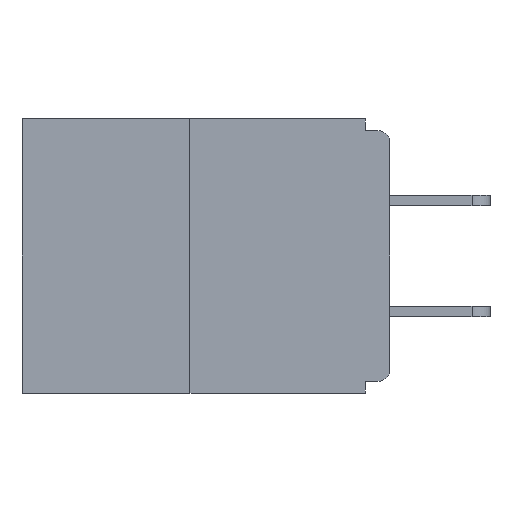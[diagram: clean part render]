
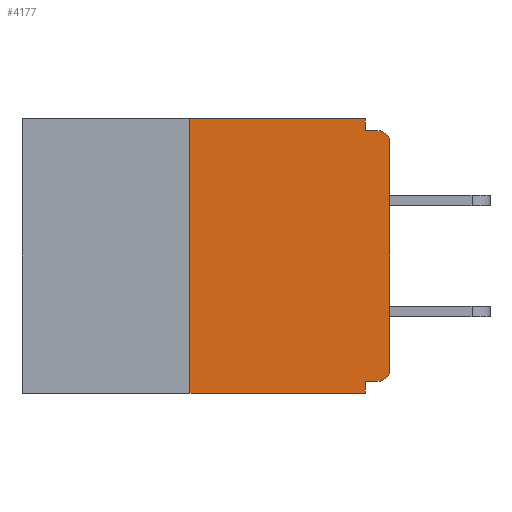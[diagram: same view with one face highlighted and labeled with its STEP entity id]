
A CAD part, left-side view. The second image highlights one B-rep face of the part: STEP entity #4177.
In plain terms, the highlighted planar face has unit normal (-1, 0, 0).
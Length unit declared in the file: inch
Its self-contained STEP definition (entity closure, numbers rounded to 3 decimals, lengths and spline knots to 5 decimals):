
#1193 = CARTESIAN_POINT ( 'NONE',  ( 0., 0., -0.03 ) ) ;
#1812 = ORIENTED_EDGE ( 'NONE', *, *, #10412, .F. ) ;
#1840 = CARTESIAN_POINT ( 'NONE',  ( 0., 0.015, -0.313 ) ) ;
#2341 = ORIENTED_EDGE ( 'NONE', *, *, #2377, .T. ) ;
#2377 = EDGE_CURVE ( 'NONE', #23291, #9017, #26616, .T. ) ;
#2640 = VERTEX_POINT ( 'NONE', #28057 ) ;
#2755 = CARTESIAN_POINT ( 'NONE',  ( 0., 0.015, -0.328 ) ) ;
#3317 = CARTESIAN_POINT ( 'NONE',  ( 0., 0., 0. ) ) ;
#4077 = EDGE_CURVE ( 'NONE', #2640, #22003, #6474, .T. ) ;
#4101 = VECTOR ( 'NONE', #17891, 39.37008 ) ;
#4158 = EDGE_CURVE ( 'NONE', #27172, #19350, #8565, .T. ) ;
#4177 = ADVANCED_FACE ( 'NONE', ( #21553 ), #20352, .F. ) ;
#4970 = DIRECTION ( 'NONE',  ( 1., 0., 0. ) ) ;
#5453 = AXIS2_PLACEMENT_3D ( 'NONE', #19837, #22134, #21942 ) ;
#5956 = CARTESIAN_POINT ( 'NONE',  ( 0., 0.031, -0.343 ) ) ;
#6432 = CARTESIAN_POINT ( 'NONE',  ( 0., 0.46, -0.343 ) ) ;
#6433 = CARTESIAN_POINT ( 'NONE',  ( 0., 0.25, -0.343 ) ) ;
#6474 = LINE ( 'NONE', #15413, #4101 ) ;
#6883 = VERTEX_POINT ( 'NONE', #27570 ) ;
#7820 = EDGE_CURVE ( 'NONE', #22003, #11822, #25873, .T. ) ;
#8263 = CARTESIAN_POINT ( 'NONE',  ( 0., 0.25, 0. ) ) ;
#8565 = LINE ( 'NONE', #24742, #20843 ) ;
#9017 = VERTEX_POINT ( 'NONE', #1193 ) ;
#9279 = EDGE_LOOP ( 'NONE', ( #1812, #12189, #24222, #17299, #24160, #23265, #2341, #11851, #18490, #23466 ) ) ;
#9849 = DIRECTION ( 'NONE',  ( 0., 0., 1. ) ) ;
#9926 = AXIS2_PLACEMENT_3D ( 'NONE', #1840, #28099, #16939 ) ;
#10339 = EDGE_CURVE ( 'NONE', #19350, #15216, #11248, .T. ) ;
#10412 = EDGE_CURVE ( 'NONE', #6883, #2640, #10582, .T. ) ;
#10576 = DIRECTION ( 'NONE',  ( 0., 0., 1. ) ) ;
#10582 = LINE ( 'NONE', #16785, #22826 ) ;
#11148 = CARTESIAN_POINT ( 'NONE',  ( 0., 0.015, -0.015 ) ) ;
#11165 = DIRECTION ( 'NONE',  ( 0., -1., 0. ) ) ;
#11248 = LINE ( 'NONE', #5956, #26266 ) ;
#11689 = DIRECTION ( 'NONE',  ( 0., 1., 0. ) ) ;
#11822 = VERTEX_POINT ( 'NONE', #11148 ) ;
#11851 = ORIENTED_EDGE ( 'NONE', *, *, #23563, .T. ) ;
#11896 = CARTESIAN_POINT ( 'NONE',  ( 0., 0.031, -0.343 ) ) ;
#11926 = VECTOR ( 'NONE', #9849, 39.37008 ) ;
#12189 = ORIENTED_EDGE ( 'NONE', *, *, #20398, .F. ) ;
#12472 = DIRECTION ( 'NONE',  ( 0., -1., 0. ) ) ;
#13795 = EDGE_CURVE ( 'NONE', #27754, #15216, #23717, .T. ) ;
#14687 = DIRECTION ( 'NONE',  ( 0., 0., -1. ) ) ;
#15216 = VERTEX_POINT ( 'NONE', #11896 ) ;
#15413 = CARTESIAN_POINT ( 'NONE',  ( 0., 0.031, 0. ) ) ;
#16361 = CARTESIAN_POINT ( 'NONE',  ( 0., 0.031, -0.328 ) ) ;
#16785 = CARTESIAN_POINT ( 'NONE',  ( 0., 0.46, 0. ) ) ;
#16939 = DIRECTION ( 'NONE',  ( 0., 0., -1. ) ) ;
#17299 = ORIENTED_EDGE ( 'NONE', *, *, #10339, .F. ) ;
#17891 = DIRECTION ( 'NONE',  ( 0., 0., -1. ) ) ;
#17924 = CARTESIAN_POINT ( 'NONE',  ( 0., 0.031, -0.015 ) ) ;
#18355 = CIRCLE ( 'NONE', #5453, 0.015 ) ;
#18490 = ORIENTED_EDGE ( 'NONE', *, *, #7820, .F. ) ;
#18917 = LINE ( 'NONE', #8263, #19923 ) ;
#19350 = VERTEX_POINT ( 'NONE', #16361 ) ;
#19837 = CARTESIAN_POINT ( 'NONE',  ( 0., 0.015, -0.03 ) ) ;
#19923 = VECTOR ( 'NONE', #10576, 39.37008 ) ;
#20015 = VECTOR ( 'NONE', #12472, 39.37008 ) ;
#20352 = PLANE ( 'NONE',  #26386 ) ;
#20398 = EDGE_CURVE ( 'NONE', #27754, #6883, #18917, .T. ) ;
#20843 = VECTOR ( 'NONE', #11689, 39.37008 ) ;
#21441 = CARTESIAN_POINT ( 'NONE',  ( 0., 0., -0.015 ) ) ;
#21553 = FACE_OUTER_BOUND ( 'NONE', #9279, .T. ) ;
#21928 = CARTESIAN_POINT ( 'NONE',  ( 0., 0., -0.313 ) ) ;
#21942 = DIRECTION ( 'NONE',  ( 0., 0., -1. ) ) ;
#22003 = VERTEX_POINT ( 'NONE', #17924 ) ;
#22134 = DIRECTION ( 'NONE',  ( -1., 0., 0. ) ) ;
#22453 = DIRECTION ( 'NONE',  ( 0., 0., -1. ) ) ;
#22826 = VECTOR ( 'NONE', #27375, 39.37008 ) ;
#22994 = VECTOR ( 'NONE', #11165, 39.37008 ) ;
#23265 = ORIENTED_EDGE ( 'NONE', *, *, #25988, .T. ) ;
#23291 = VERTEX_POINT ( 'NONE', #21928 ) ;
#23466 = ORIENTED_EDGE ( 'NONE', *, *, #4077, .F. ) ;
#23563 = EDGE_CURVE ( 'NONE', #9017, #11822, #18355, .T. ) ;
#23717 = LINE ( 'NONE', #6432, #22994 ) ;
#24160 = ORIENTED_EDGE ( 'NONE', *, *, #4158, .F. ) ;
#24222 = ORIENTED_EDGE ( 'NONE', *, *, #13795, .T. ) ;
#24376 = CARTESIAN_POINT ( 'NONE',  ( 0., 0.46, 0. ) ) ;
#24742 = CARTESIAN_POINT ( 'NONE',  ( 0., 0., -0.328 ) ) ;
#25873 = LINE ( 'NONE', #21441, #20015 ) ;
#25988 = EDGE_CURVE ( 'NONE', #27172, #23291, #26154, .T. ) ;
#26154 = CIRCLE ( 'NONE', #9926, 0.015 ) ;
#26266 = VECTOR ( 'NONE', #14687, 39.37008 ) ;
#26386 = AXIS2_PLACEMENT_3D ( 'NONE', #24376, #4970, #22453 ) ;
#26616 = LINE ( 'NONE', #3317, #11926 ) ;
#27172 = VERTEX_POINT ( 'NONE', #2755 ) ;
#27375 = DIRECTION ( 'NONE',  ( 0., -1., 0. ) ) ;
#27570 = CARTESIAN_POINT ( 'NONE',  ( 0., 0.25, 0. ) ) ;
#27754 = VERTEX_POINT ( 'NONE', #6433 ) ;
#28057 = CARTESIAN_POINT ( 'NONE',  ( 0., 0.031, 0. ) ) ;
#28099 = DIRECTION ( 'NONE',  ( -1., 0., 0. ) ) ;
